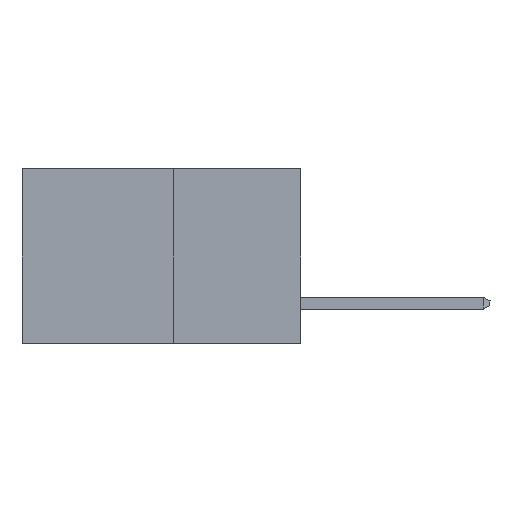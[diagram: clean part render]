
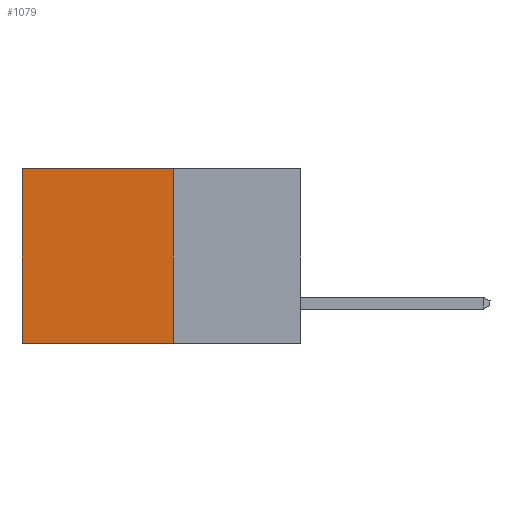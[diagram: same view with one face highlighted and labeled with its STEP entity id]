
A CAD part, left-side view. The second image highlights one B-rep face of the part: STEP entity #1079.
In plain terms, the highlighted planar face has unit normal (-1, 0, 0).
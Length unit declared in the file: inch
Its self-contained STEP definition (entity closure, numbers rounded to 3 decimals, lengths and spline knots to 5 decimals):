
#197 = LINE ( 'NONE', #5285, #2062 ) ;
#450 = VERTEX_POINT ( 'NONE', #7160 ) ;
#1079 = ADVANCED_FACE ( 'NONE', ( #7414 ), #5679, .F. ) ;
#1311 = LINE ( 'NONE', #5557, #2981 ) ;
#1907 = DIRECTION ( 'NONE',  ( 0., 0., -1. ) ) ;
#2062 = VECTOR ( 'NONE', #5122, 39.37008 ) ;
#2344 = EDGE_CURVE ( 'NONE', #7597, #6148, #1311, .T. ) ;
#2433 = DIRECTION ( 'NONE',  ( 1., 0., 0. ) ) ;
#2499 = DIRECTION ( 'NONE',  ( 0., 0., -1. ) ) ;
#2705 = EDGE_CURVE ( 'NONE', #6148, #450, #5887, .T. ) ;
#2977 = EDGE_LOOP ( 'NONE', ( #3928, #3931, #3941, #3944 ) ) ;
#2981 = VECTOR ( 'NONE', #3567, 39.37008 ) ;
#3108 = AXIS2_PLACEMENT_3D ( 'NONE', #5676, #2433, #2499 ) ;
#3337 = CARTESIAN_POINT ( 'NONE',  ( 0.277, 0.27, -0.37 ) ) ;
#3553 = CARTESIAN_POINT ( 'NONE',  ( 0.277, 0.27, 0. ) ) ;
#3560 = VERTEX_POINT ( 'NONE', #3337 ) ;
#3567 = DIRECTION ( 'NONE',  ( 0., 1., 0. ) ) ;
#3928 = ORIENTED_EDGE ( 'NONE', *, *, #2705, .T. ) ;
#3931 = ORIENTED_EDGE ( 'NONE', *, *, #5379, .F. ) ;
#3941 = ORIENTED_EDGE ( 'NONE', *, *, #6346, .F. ) ;
#3944 = ORIENTED_EDGE ( 'NONE', *, *, #2344, .T. ) ;
#4362 = CARTESIAN_POINT ( 'NONE',  ( 0.277, 0.59, 0. ) ) ;
#5122 = DIRECTION ( 'NONE',  ( 0., 1., 0. ) ) ;
#5285 = CARTESIAN_POINT ( 'NONE',  ( 0.277, 0.27, -0.37 ) ) ;
#5379 = EDGE_CURVE ( 'NONE', #3560, #450, #197, .T. ) ;
#5557 = CARTESIAN_POINT ( 'NONE',  ( 0.277, 0.27, 0. ) ) ;
#5676 = CARTESIAN_POINT ( 'NONE',  ( 0.277, 0.27, -0.37 ) ) ;
#5679 = PLANE ( 'NONE',  #3108 ) ;
#5887 = LINE ( 'NONE', #8484, #7272 ) ;
#6009 = VECTOR ( 'NONE', #8508, 39.37008 ) ;
#6148 = VERTEX_POINT ( 'NONE', #4362 ) ;
#6198 = LINE ( 'NONE', #8430, #6009 ) ;
#6346 = EDGE_CURVE ( 'NONE', #7597, #3560, #6198, .T. ) ;
#7160 = CARTESIAN_POINT ( 'NONE',  ( 0.277, 0.59, -0.37 ) ) ;
#7272 = VECTOR ( 'NONE', #1907, 39.37008 ) ;
#7414 = FACE_OUTER_BOUND ( 'NONE', #2977, .T. ) ;
#7597 = VERTEX_POINT ( 'NONE', #3553 ) ;
#8430 = CARTESIAN_POINT ( 'NONE',  ( 0.277, 0.27, -0.37 ) ) ;
#8484 = CARTESIAN_POINT ( 'NONE',  ( 0.277, 0.59, -0.37 ) ) ;
#8508 = DIRECTION ( 'NONE',  ( 0., 0., -1. ) ) ;
